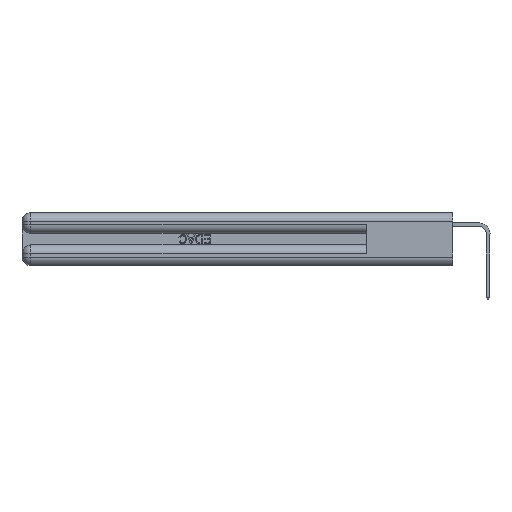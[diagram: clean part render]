
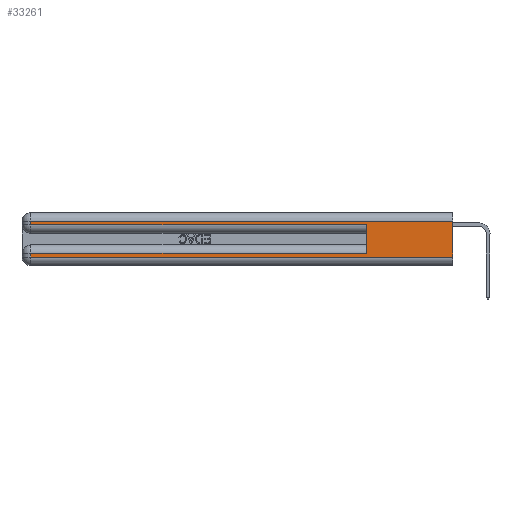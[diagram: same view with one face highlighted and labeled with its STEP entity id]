
A CAD part, left-side view. The second image highlights one B-rep face of the part: STEP entity #33261.
In plain terms, the highlighted planar face has unit normal (-1, 0, 0).
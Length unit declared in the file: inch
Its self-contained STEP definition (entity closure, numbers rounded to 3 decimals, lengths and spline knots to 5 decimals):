
#129 = DIRECTION ( 'NONE',  ( 0., 0., 1. ) ) ;
#238 = EDGE_CURVE ( 'NONE', #34912, #32825, #38115, .T. ) ;
#530 = DIRECTION ( 'NONE',  ( 0., 0., -1. ) ) ;
#565 = VECTOR ( 'NONE', #5215, 39.37008 ) ;
#2000 = CARTESIAN_POINT ( 'NONE',  ( 0., 0., 0.06 ) ) ;
#4130 = FACE_OUTER_BOUND ( 'NONE', #30256, .T. ) ;
#5196 = DIRECTION ( 'NONE',  ( 0., -1., 0. ) ) ;
#5215 = DIRECTION ( 'NONE',  ( 0., 1., 0. ) ) ;
#7580 = EDGE_CURVE ( 'NONE', #36258, #32825, #39225, .T. ) ;
#7631 = VECTOR ( 'NONE', #129, 39.37008 ) ;
#7668 = DIRECTION ( 'NONE',  ( 1., 0., 0. ) ) ;
#8658 = VERTEX_POINT ( 'NONE', #20565 ) ;
#8713 = CARTESIAN_POINT ( 'NONE',  ( 0., 2.94, 0.31 ) ) ;
#8898 = LINE ( 'NONE', #20790, #565 ) ;
#9621 = ORIENTED_EDGE ( 'NONE', *, *, #38293, .T. ) ;
#9640 = CARTESIAN_POINT ( 'NONE',  ( 0., 0., 0.285 ) ) ;
#9663 = ORIENTED_EDGE ( 'NONE', *, *, #34885, .T. ) ;
#9733 = CARTESIAN_POINT ( 'NONE',  ( 0., 2.94, 0.085 ) ) ;
#10363 = VECTOR ( 'NONE', #34792, 39.37008 ) ;
#11468 = CARTESIAN_POINT ( 'NONE',  ( 0., 0., 0.31 ) ) ;
#12293 = EDGE_CURVE ( 'NONE', #40536, #16086, #12614, .T. ) ;
#12614 = LINE ( 'NONE', #25492, #36640 ) ;
#13951 = CARTESIAN_POINT ( 'NONE',  ( 0., 0., 0.37 ) ) ;
#15483 = ORIENTED_EDGE ( 'NONE', *, *, #25711, .F. ) ;
#15929 = LINE ( 'NONE', #31394, #7631 ) ;
#16086 = VERTEX_POINT ( 'NONE', #30359 ) ;
#16927 = PLANE ( 'NONE',  #18515 ) ;
#17788 = CARTESIAN_POINT ( 'NONE',  ( 0., 0., 0.06 ) ) ;
#18107 = VERTEX_POINT ( 'NONE', #29988 ) ;
#18378 = ORIENTED_EDGE ( 'NONE', *, *, #12293, .T. ) ;
#18515 = AXIS2_PLACEMENT_3D ( 'NONE', #20109, #7668, #29578 ) ;
#19497 = LINE ( 'NONE', #38337, #24938 ) ;
#19655 = LINE ( 'NONE', #37922, #10363 ) ;
#20109 = CARTESIAN_POINT ( 'NONE',  ( 0., 0., 0.37 ) ) ;
#20460 = ORIENTED_EDGE ( 'NONE', *, *, #22288, .T. ) ;
#20565 = CARTESIAN_POINT ( 'NONE',  ( 0., 0.6, 0.085 ) ) ;
#20790 = CARTESIAN_POINT ( 'NONE',  ( 0., 0., 0.085 ) ) ;
#21460 = VECTOR ( 'NONE', #31892, 39.37008 ) ;
#22288 = EDGE_CURVE ( 'NONE', #36424, #36258, #19655, .T. ) ;
#22729 = DIRECTION ( 'NONE',  ( 0., 1., 0. ) ) ;
#23806 = LINE ( 'NONE', #9640, #31174 ) ;
#23815 = ORIENTED_EDGE ( 'NONE', *, *, #24141, .T. ) ;
#24141 = EDGE_CURVE ( 'NONE', #34912, #40536, #19497, .T. ) ;
#24938 = VECTOR ( 'NONE', #22729, 39.37008 ) ;
#25492 = CARTESIAN_POINT ( 'NONE',  ( 0., 2.94, 0.37 ) ) ;
#25711 = EDGE_CURVE ( 'NONE', #8658, #18107, #15929, .T. ) ;
#27236 = ORIENTED_EDGE ( 'NONE', *, *, #238, .F. ) ;
#29578 = DIRECTION ( 'NONE',  ( 0., 0., -1. ) ) ;
#29988 = CARTESIAN_POINT ( 'NONE',  ( 0., 0.6, 0.285 ) ) ;
#30256 = EDGE_LOOP ( 'NONE', ( #27236, #23815, #18378, #9621, #15483, #9663, #20460, #33728 ) ) ;
#30359 = CARTESIAN_POINT ( 'NONE',  ( 0., 2.94, 0.285 ) ) ;
#30707 = CARTESIAN_POINT ( 'NONE',  ( 0., 2.94, 0.06 ) ) ;
#30928 = VECTOR ( 'NONE', #5196, 39.37008 ) ;
#31174 = VECTOR ( 'NONE', #37852, 39.37008 ) ;
#31394 = CARTESIAN_POINT ( 'NONE',  ( 0., 0.6, 0.145 ) ) ;
#31892 = DIRECTION ( 'NONE',  ( 0., 0., -1. ) ) ;
#32825 = VERTEX_POINT ( 'NONE', #17788 ) ;
#33261 = ADVANCED_FACE ( 'NONE', ( #4130 ), #16927, .F. ) ;
#33728 = ORIENTED_EDGE ( 'NONE', *, *, #7580, .T. ) ;
#34792 = DIRECTION ( 'NONE',  ( 0., 0., -1. ) ) ;
#34885 = EDGE_CURVE ( 'NONE', #8658, #36424, #8898, .T. ) ;
#34912 = VERTEX_POINT ( 'NONE', #11468 ) ;
#36258 = VERTEX_POINT ( 'NONE', #30707 ) ;
#36424 = VERTEX_POINT ( 'NONE', #9733 ) ;
#36640 = VECTOR ( 'NONE', #530, 39.37008 ) ;
#37852 = DIRECTION ( 'NONE',  ( 0., -1., 0. ) ) ;
#37922 = CARTESIAN_POINT ( 'NONE',  ( 0., 2.94, 0.37 ) ) ;
#38115 = LINE ( 'NONE', #13951, #21460 ) ;
#38293 = EDGE_CURVE ( 'NONE', #16086, #18107, #23806, .T. ) ;
#38337 = CARTESIAN_POINT ( 'NONE',  ( 0., 0., 0.31 ) ) ;
#39225 = LINE ( 'NONE', #2000, #30928 ) ;
#40536 = VERTEX_POINT ( 'NONE', #8713 ) ;
